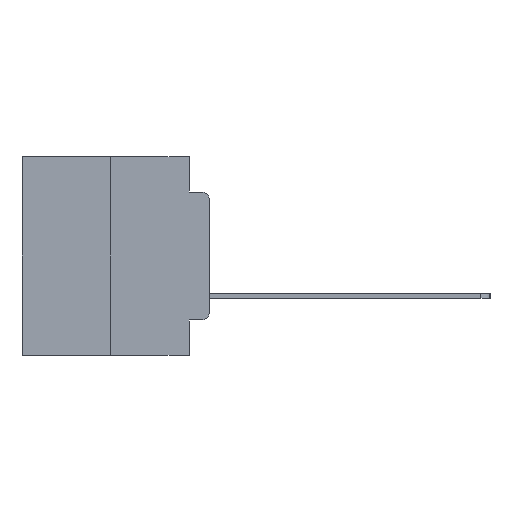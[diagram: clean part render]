
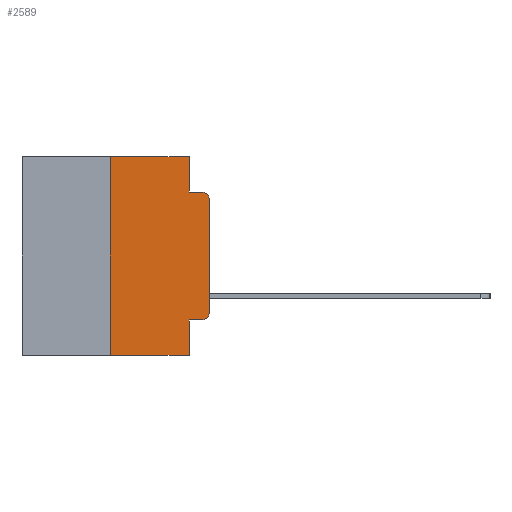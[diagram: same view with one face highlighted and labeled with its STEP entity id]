
A CAD part, left-side view. The second image highlights one B-rep face of the part: STEP entity #2589.
In plain terms, the highlighted planar face has unit normal (-1, 0, 0).
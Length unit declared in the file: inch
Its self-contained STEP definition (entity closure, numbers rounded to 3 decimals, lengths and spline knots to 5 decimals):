
#414 = EDGE_CURVE ( 'NONE', #14646, #21628, #3381, .T. ) ;
#536 = ORIENTED_EDGE ( 'NONE', *, *, #24818, .T. ) ;
#998 = CARTESIAN_POINT ( 'NONE',  ( 0., 0.051, -0.0885 ) ) ;
#1460 = CARTESIAN_POINT ( 'NONE',  ( 0., 0.051, -0.4115 ) ) ;
#1633 = DIRECTION ( 'NONE',  ( 1., 0., 0. ) ) ;
#1719 = EDGE_CURVE ( 'NONE', #4005, #8277, #2997, .T. ) ;
#1761 = CARTESIAN_POINT ( 'NONE',  ( 0., 0.473, 0. ) ) ;
#1776 = ORIENTED_EDGE ( 'NONE', *, *, #6525, .F. ) ;
#2372 = LINE ( 'NONE', #9401, #23631 ) ;
#2512 = VECTOR ( 'NONE', #13533, 39.37008 ) ;
#2589 = ADVANCED_FACE ( 'NONE', ( #15587 ), #4697, .F. ) ;
#2981 = VERTEX_POINT ( 'NONE', #1460 ) ;
#2997 = CIRCLE ( 'NONE', #8179, 0.02 ) ;
#3147 = EDGE_CURVE ( 'NONE', #20108, #4005, #23783, .T. ) ;
#3381 = LINE ( 'NONE', #6077, #24583 ) ;
#3605 = ORIENTED_EDGE ( 'NONE', *, *, #3147, .T. ) ;
#3906 = DIRECTION ( 'NONE',  ( 0., 0., -1. ) ) ;
#4005 = VERTEX_POINT ( 'NONE', #14147 ) ;
#4394 = ORIENTED_EDGE ( 'NONE', *, *, #1719, .T. ) ;
#4478 = DIRECTION ( 'NONE',  ( 0., 0., -1. ) ) ;
#4697 = PLANE ( 'NONE',  #26216 ) ;
#5162 = VERTEX_POINT ( 'NONE', #14763 ) ;
#5225 = VECTOR ( 'NONE', #22940, 39.37008 ) ;
#6077 = CARTESIAN_POINT ( 'NONE',  ( 0., 0.473, 0. ) ) ;
#6397 = ORIENTED_EDGE ( 'NONE', *, *, #17606, .F. ) ;
#6487 = DIRECTION ( 'NONE',  ( 0., 0., -1. ) ) ;
#6521 = DIRECTION ( 'NONE',  ( -1., 0., 0. ) ) ;
#6525 = EDGE_CURVE ( 'NONE', #2981, #5162, #2372, .T. ) ;
#6600 = ORIENTED_EDGE ( 'NONE', *, *, #14841, .F. ) ;
#6751 = CIRCLE ( 'NONE', #21562, 0.02 ) ;
#6792 = CARTESIAN_POINT ( 'NONE',  ( 0., 0., -0.3915 ) ) ;
#7576 = VECTOR ( 'NONE', #20119, 39.37008 ) ;
#7855 = CARTESIAN_POINT ( 'NONE',  ( 0., 0.051, 0. ) ) ;
#8179 = AXIS2_PLACEMENT_3D ( 'NONE', #8614, #6521, #6487 ) ;
#8231 = LINE ( 'NONE', #22116, #7576 ) ;
#8277 = VERTEX_POINT ( 'NONE', #10293 ) ;
#8291 = DIRECTION ( 'NONE',  ( 0., 0., -1. ) ) ;
#8330 = ORIENTED_EDGE ( 'NONE', *, *, #19467, .T. ) ;
#8438 = DIRECTION ( 'NONE',  ( 0., -1., 0. ) ) ;
#8614 = CARTESIAN_POINT ( 'NONE',  ( 0., 0.02, -0.1085 ) ) ;
#8791 = EDGE_CURVE ( 'NONE', #12272, #5162, #10479, .T. ) ;
#9401 = CARTESIAN_POINT ( 'NONE',  ( 0., 0.051, 0. ) ) ;
#9827 = VECTOR ( 'NONE', #16036, 39.37008 ) ;
#10293 = CARTESIAN_POINT ( 'NONE',  ( 0., 0.02, -0.0885 ) ) ;
#10479 = LINE ( 'NONE', #13957, #9827 ) ;
#10731 = LINE ( 'NONE', #22855, #5225 ) ;
#11383 = CARTESIAN_POINT ( 'NONE',  ( 0., 0.02, -0.3915 ) ) ;
#11986 = VERTEX_POINT ( 'NONE', #12039 ) ;
#12039 = CARTESIAN_POINT ( 'NONE',  ( 0., 0.02, -0.4115 ) ) ;
#12048 = EDGE_CURVE ( 'NONE', #12272, #14646, #23100, .T. ) ;
#12272 = VERTEX_POINT ( 'NONE', #23156 ) ;
#13104 = VECTOR ( 'NONE', #3906, 39.37008 ) ;
#13442 = DIRECTION ( 'NONE',  ( 0., 0., -1. ) ) ;
#13533 = DIRECTION ( 'NONE',  ( 0., 0., 1. ) ) ;
#13597 = CARTESIAN_POINT ( 'NONE',  ( 0., 0., 0. ) ) ;
#13957 = CARTESIAN_POINT ( 'NONE',  ( 0., 0.473, -0.5 ) ) ;
#14147 = CARTESIAN_POINT ( 'NONE',  ( 0., 0., -0.1085 ) ) ;
#14347 = EDGE_LOOP ( 'NONE', ( #3605, #4394, #6397, #6600, #15967, #17824, #21418, #1776, #536, #8330 ) ) ;
#14646 = VERTEX_POINT ( 'NONE', #15716 ) ;
#14763 = CARTESIAN_POINT ( 'NONE',  ( 0., 0.051, -0.5 ) ) ;
#14841 = EDGE_CURVE ( 'NONE', #21628, #16764, #23925, .T. ) ;
#15587 = FACE_OUTER_BOUND ( 'NONE', #14347, .T. ) ;
#15716 = CARTESIAN_POINT ( 'NONE',  ( 0., 0.25, 0. ) ) ;
#15967 = ORIENTED_EDGE ( 'NONE', *, *, #414, .F. ) ;
#16036 = DIRECTION ( 'NONE',  ( 0., -1., 0. ) ) ;
#16764 = VERTEX_POINT ( 'NONE', #998 ) ;
#17606 = EDGE_CURVE ( 'NONE', #16764, #8277, #10731, .T. ) ;
#17773 = VECTOR ( 'NONE', #24485, 39.37008 ) ;
#17824 = ORIENTED_EDGE ( 'NONE', *, *, #12048, .F. ) ;
#18437 = CARTESIAN_POINT ( 'NONE',  ( 0., 0.051, 0. ) ) ;
#19467 = EDGE_CURVE ( 'NONE', #11986, #20108, #6751, .T. ) ;
#20108 = VERTEX_POINT ( 'NONE', #6792 ) ;
#20119 = DIRECTION ( 'NONE',  ( 0., -1., 0. ) ) ;
#21418 = ORIENTED_EDGE ( 'NONE', *, *, #8791, .T. ) ;
#21562 = AXIS2_PLACEMENT_3D ( 'NONE', #11383, #25579, #13442 ) ;
#21628 = VERTEX_POINT ( 'NONE', #7855 ) ;
#22116 = CARTESIAN_POINT ( 'NONE',  ( 0., 0.051, -0.4115 ) ) ;
#22855 = CARTESIAN_POINT ( 'NONE',  ( 0., 0.051, -0.0885 ) ) ;
#22940 = DIRECTION ( 'NONE',  ( 0., -1., 0. ) ) ;
#23100 = LINE ( 'NONE', #24400, #17773 ) ;
#23156 = CARTESIAN_POINT ( 'NONE',  ( 0., 0.25, -0.5 ) ) ;
#23631 = VECTOR ( 'NONE', #8291, 39.37008 ) ;
#23783 = LINE ( 'NONE', #13597, #2512 ) ;
#23925 = LINE ( 'NONE', #18437, #13104 ) ;
#24400 = CARTESIAN_POINT ( 'NONE',  ( 0., 0.25, 0. ) ) ;
#24485 = DIRECTION ( 'NONE',  ( 0., 0., 1. ) ) ;
#24583 = VECTOR ( 'NONE', #8438, 39.37008 ) ;
#24818 = EDGE_CURVE ( 'NONE', #2981, #11986, #8231, .T. ) ;
#25579 = DIRECTION ( 'NONE',  ( -1., 0., 0. ) ) ;
#26216 = AXIS2_PLACEMENT_3D ( 'NONE', #1761, #1633, #4478 ) ;
